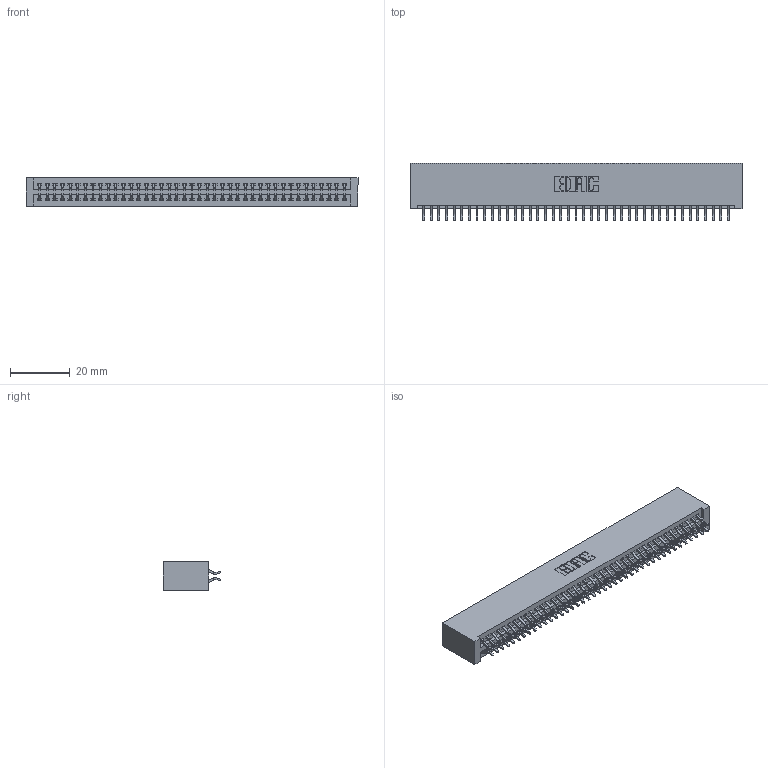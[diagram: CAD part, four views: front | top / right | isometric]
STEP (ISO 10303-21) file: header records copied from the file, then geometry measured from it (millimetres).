
FILE_DESCRIPTION (( 'STEP AP203' ), '1' );
FILE_NAME ('345-082-556-201.STEP', '2018-10-03T23:05:56', ( '' ), ( '' ), 'SwSTEP 2.0', 'SolidWorks 2016', '' );
FILE_SCHEMA (( 'CONFIG_CONTROL_DESIGN' ));
Length unit declared in the file: inch
Products named in the file (3): 345 Part_No Mounting Lugs; 345-292-001_556 Tail; 345-082-556-201
Assembly tree (83 placements, depth 2):
  345-082-556-201
    345 Part_No Mounting Lugs
    345-292-001_556 Tail  x82
Bounding box: 110.74 x 19.24 x 9.4 mm (x, y, z)
Volume: 11361.2 mm3; surface area: 17005.8 mm2
Topology: 83 solids, 83 shells, 4710 faces, 14011 edges, 9230 vertices
Faces by surface type: plane 3110, cylinder 1600
Entity records: 32247 total; most frequent: CARTESIAN_POINT 5420, ORIENTED_EDGE 5342, DIRECTION 4763, EDGE_CURVE 2671, LINE 2375, VECTOR 2375, VERTEX_POINT 1778, AXIS2_PLACEMENT_3D 1194
